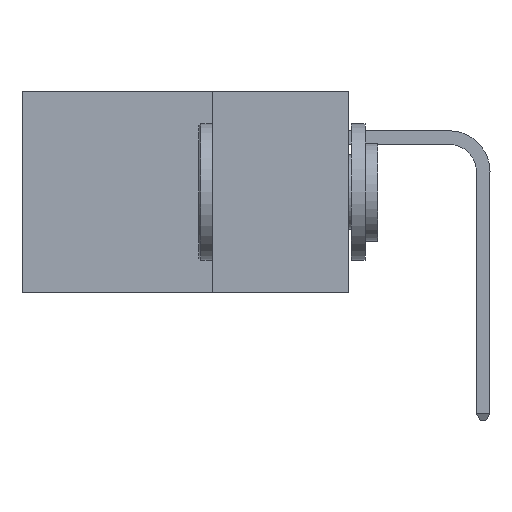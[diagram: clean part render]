
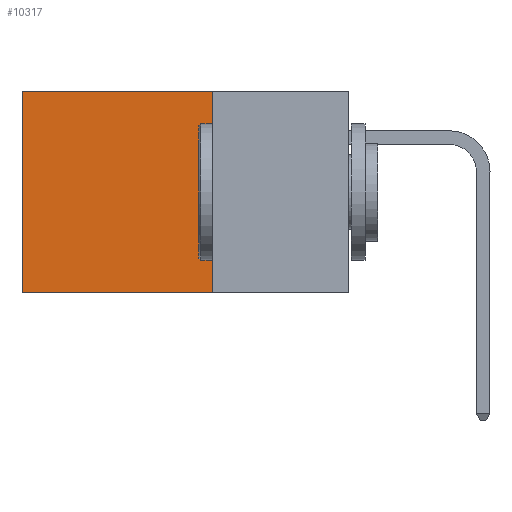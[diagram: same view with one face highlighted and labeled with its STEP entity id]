
A CAD part, left-side view. The second image highlights one B-rep face of the part: STEP entity #10317.
In plain terms, the highlighted planar face has unit normal (-1, 0, 0).
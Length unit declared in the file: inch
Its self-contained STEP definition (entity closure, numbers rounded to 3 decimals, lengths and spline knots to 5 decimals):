
#577 = CARTESIAN_POINT ( 'NONE',  ( 0.2875, 0.25, 0. ) ) ;
#853 = EDGE_CURVE ( 'NONE', #6033, #26570, #19669, .T. ) ;
#1333 = EDGE_LOOP ( 'NONE', ( #15455, #4017, #1999, #14392 ) ) ;
#1999 = ORIENTED_EDGE ( 'NONE', *, *, #24063, .F. ) ;
#2097 = EDGE_CURVE ( 'NONE', #17482, #21926, #24558, .T. ) ;
#4017 = ORIENTED_EDGE ( 'NONE', *, *, #853, .F. ) ;
#4236 = CARTESIAN_POINT ( 'NONE',  ( 0.2875, 0.25, 0. ) ) ;
#4622 = CARTESIAN_POINT ( 'NONE',  ( 0.2875, 0.6, 0. ) ) ;
#4968 = DIRECTION ( 'NONE',  ( 1., 0., 0. ) ) ;
#6033 = VERTEX_POINT ( 'NONE', #17803 ) ;
#8464 = VECTOR ( 'NONE', #16152, 39.37008 ) ;
#8791 = VECTOR ( 'NONE', #18745, 39.37008 ) ;
#9648 = DIRECTION ( 'NONE',  ( 0., 1., 0. ) ) ;
#10317 = ADVANCED_FACE ( 'NONE', ( #25049 ), #17599, .F. ) ;
#13391 = CARTESIAN_POINT ( 'NONE',  ( 0.2875, 0.6, 0. ) ) ;
#13890 = CARTESIAN_POINT ( 'NONE',  ( 0.2875, 0.25, 0. ) ) ;
#14392 = ORIENTED_EDGE ( 'NONE', *, *, #2097, .T. ) ;
#15185 = VECTOR ( 'NONE', #25926, 39.37008 ) ;
#15225 = EDGE_CURVE ( 'NONE', #21926, #26570, #15825, .T. ) ;
#15455 = ORIENTED_EDGE ( 'NONE', *, *, #15225, .T. ) ;
#15566 = CARTESIAN_POINT ( 'NONE',  ( 0.2875, 0.25, -0.37 ) ) ;
#15825 = LINE ( 'NONE', #13391, #15185 ) ;
#16152 = DIRECTION ( 'NONE',  ( 0., 1., 0. ) ) ;
#16611 = CARTESIAN_POINT ( 'NONE',  ( 0.2875, 0.25, 0. ) ) ;
#17482 = VERTEX_POINT ( 'NONE', #4236 ) ;
#17599 = PLANE ( 'NONE',  #17931 ) ;
#17803 = CARTESIAN_POINT ( 'NONE',  ( 0.2875, 0.25, -0.37 ) ) ;
#17931 = AXIS2_PLACEMENT_3D ( 'NONE', #577, #4968, #19750 ) ;
#18745 = DIRECTION ( 'NONE',  ( 0., 0., -1. ) ) ;
#19669 = LINE ( 'NONE', #15566, #8464 ) ;
#19750 = DIRECTION ( 'NONE',  ( 0., 0., -1. ) ) ;
#19990 = LINE ( 'NONE', #16611, #8791 ) ;
#21926 = VERTEX_POINT ( 'NONE', #4622 ) ;
#23455 = CARTESIAN_POINT ( 'NONE',  ( 0.2875, 0.6, -0.37 ) ) ;
#23908 = VECTOR ( 'NONE', #9648, 39.37008 ) ;
#24063 = EDGE_CURVE ( 'NONE', #17482, #6033, #19990, .T. ) ;
#24558 = LINE ( 'NONE', #13890, #23908 ) ;
#25049 = FACE_OUTER_BOUND ( 'NONE', #1333, .T. ) ;
#25926 = DIRECTION ( 'NONE',  ( 0., 0., -1. ) ) ;
#26570 = VERTEX_POINT ( 'NONE', #23455 ) ;
